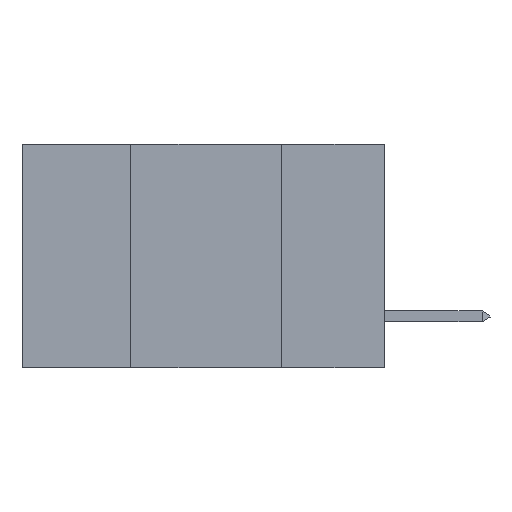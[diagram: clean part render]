
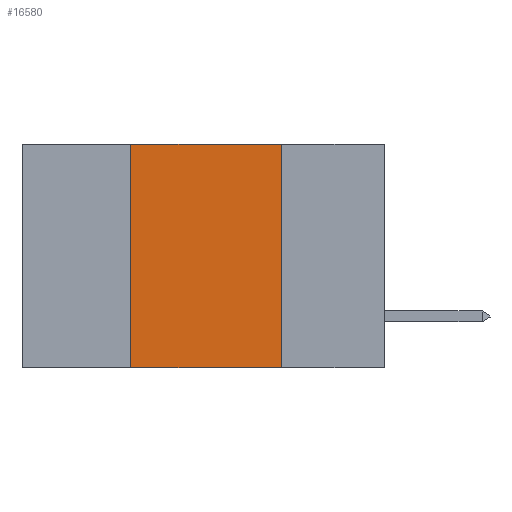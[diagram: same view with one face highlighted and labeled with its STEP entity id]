
A CAD part, left-side view. The second image highlights one B-rep face of the part: STEP entity #16580.
In plain terms, the highlighted planar face has unit normal (-1, 0, 0).
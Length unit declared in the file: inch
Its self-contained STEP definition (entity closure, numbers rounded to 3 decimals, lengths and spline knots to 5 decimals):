
#124 = CARTESIAN_POINT ( 'NONE',  ( 0., 0.42, 0. ) ) ;
#270 = VERTEX_POINT ( 'NONE', #2690 ) ;
#342 = VECTOR ( 'NONE', #22522, 39.37008 ) ;
#710 = CARTESIAN_POINT ( 'NONE',  ( 0., 0.17, 0. ) ) ;
#1421 = CARTESIAN_POINT ( 'NONE',  ( 0., 0.17, 0. ) ) ;
#1637 = CARTESIAN_POINT ( 'NONE',  ( 0., 0.6, -0.37 ) ) ;
#2201 = DIRECTION ( 'NONE',  ( 0., 0., -1. ) ) ;
#2690 = CARTESIAN_POINT ( 'NONE',  ( 0., 0.17, -0.37 ) ) ;
#3210 = EDGE_CURVE ( 'NONE', #23186, #15109, #20421, .T. ) ;
#4146 = ORIENTED_EDGE ( 'NONE', *, *, #19158, .T. ) ;
#4414 = VECTOR ( 'NONE', #2201, 39.37008 ) ;
#4700 = LINE ( 'NONE', #710, #4414 ) ;
#5687 = VECTOR ( 'NONE', #13341, 39.37008 ) ;
#5716 = VERTEX_POINT ( 'NONE', #11666 ) ;
#7022 = FACE_OUTER_BOUND ( 'NONE', #11230, .T. ) ;
#7771 = DIRECTION ( 'NONE',  ( 1., 0., 0. ) ) ;
#7807 = CARTESIAN_POINT ( 'NONE',  ( 0., 0.6, 0. ) ) ;
#7857 = CARTESIAN_POINT ( 'NONE',  ( 0., 0.6, 0. ) ) ;
#11230 = EDGE_LOOP ( 'NONE', ( #15378, #23370, #20730, #4146 ) ) ;
#11666 = CARTESIAN_POINT ( 'NONE',  ( 0., 0.42, -0.37 ) ) ;
#12052 = EDGE_CURVE ( 'NONE', #5716, #23186, #17457, .T. ) ;
#12579 = CARTESIAN_POINT ( 'NONE',  ( 0., 0.42, 0. ) ) ;
#13341 = DIRECTION ( 'NONE',  ( 0., -1., 0. ) ) ;
#15109 = VERTEX_POINT ( 'NONE', #1421 ) ;
#15378 = ORIENTED_EDGE ( 'NONE', *, *, #16269, .F. ) ;
#16269 = EDGE_CURVE ( 'NONE', #15109, #270, #4700, .T. ) ;
#16580 = ADVANCED_FACE ( 'NONE', ( #7022 ), #17165, .F. ) ;
#17165 = PLANE ( 'NONE',  #18376 ) ;
#17457 = LINE ( 'NONE', #12579, #342 ) ;
#17818 = LINE ( 'NONE', #1637, #19270 ) ;
#18376 = AXIS2_PLACEMENT_3D ( 'NONE', #7857, #7771, #20956 ) ;
#19158 = EDGE_CURVE ( 'NONE', #5716, #270, #17818, .T. ) ;
#19270 = VECTOR ( 'NONE', #23998, 39.37008 ) ;
#20421 = LINE ( 'NONE', #7807, #5687 ) ;
#20730 = ORIENTED_EDGE ( 'NONE', *, *, #12052, .F. ) ;
#20956 = DIRECTION ( 'NONE',  ( 0., 0., -1. ) ) ;
#22522 = DIRECTION ( 'NONE',  ( 0., 0., 1. ) ) ;
#23186 = VERTEX_POINT ( 'NONE', #124 ) ;
#23370 = ORIENTED_EDGE ( 'NONE', *, *, #3210, .F. ) ;
#23998 = DIRECTION ( 'NONE',  ( 0., -1., 0. ) ) ;
